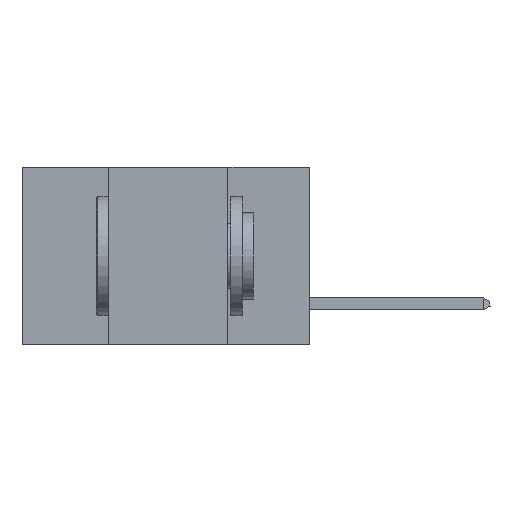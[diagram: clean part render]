
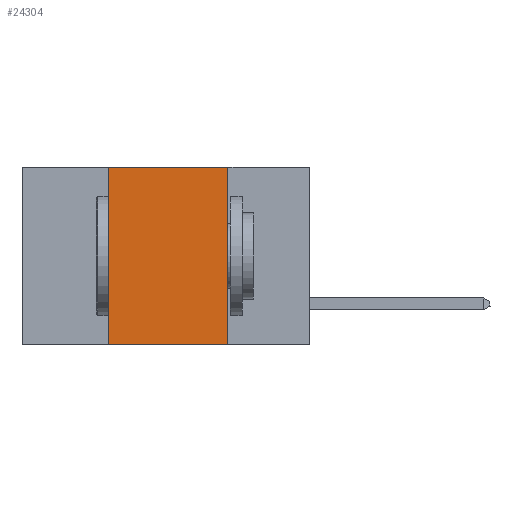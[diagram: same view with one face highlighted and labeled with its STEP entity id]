
A CAD part, left-side view. The second image highlights one B-rep face of the part: STEP entity #24304.
In plain terms, the highlighted planar face has unit normal (-1, 0, 0).
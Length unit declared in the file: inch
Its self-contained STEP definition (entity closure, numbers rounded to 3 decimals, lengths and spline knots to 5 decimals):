
#464 = AXIS2_PLACEMENT_3D ( 'NONE', #31716, #12325, #34604 ) ;
#1781 = ORIENTED_EDGE ( 'NONE', *, *, #29595, .T. ) ;
#3435 = VECTOR ( 'NONE', #9895, 39.37008 ) ;
#3680 = PLANE ( 'NONE',  #464 ) ;
#3790 = VERTEX_POINT ( 'NONE', #25234 ) ;
#9895 = DIRECTION ( 'NONE',  ( 0., -1., 0. ) ) ;
#10277 = LINE ( 'NONE', #16529, #36009 ) ;
#10820 = LINE ( 'NONE', #23432, #3435 ) ;
#10913 = ORIENTED_EDGE ( 'NONE', *, *, #31078, .F. ) ;
#11638 = LINE ( 'NONE', #31264, #20411 ) ;
#11940 = CARTESIAN_POINT ( 'NONE',  ( 0., 0.17, 0. ) ) ;
#12318 = VERTEX_POINT ( 'NONE', #19373 ) ;
#12325 = DIRECTION ( 'NONE',  ( 1., 0., 0. ) ) ;
#16529 = CARTESIAN_POINT ( 'NONE',  ( 0., 0.17, 0. ) ) ;
#16829 = EDGE_CURVE ( 'NONE', #3790, #17290, #10820, .T. ) ;
#16951 = CARTESIAN_POINT ( 'NONE',  ( 0., 0.42, -0.37 ) ) ;
#17148 = LINE ( 'NONE', #29473, #35852 ) ;
#17290 = VERTEX_POINT ( 'NONE', #11940 ) ;
#19373 = CARTESIAN_POINT ( 'NONE',  ( 0., 0.17, -0.37 ) ) ;
#20411 = VECTOR ( 'NONE', #25915, 39.37008 ) ;
#20912 = DIRECTION ( 'NONE',  ( 0., 0., 1. ) ) ;
#21212 = VERTEX_POINT ( 'NONE', #16951 ) ;
#23090 = DIRECTION ( 'NONE',  ( 0., 0., -1. ) ) ;
#23432 = CARTESIAN_POINT ( 'NONE',  ( 0., 0.6, 0. ) ) ;
#24286 = FACE_OUTER_BOUND ( 'NONE', #30659, .T. ) ;
#24304 = ADVANCED_FACE ( 'NONE', ( #24286 ), #3680, .F. ) ;
#25234 = CARTESIAN_POINT ( 'NONE',  ( 0., 0.42, 0. ) ) ;
#25915 = DIRECTION ( 'NONE',  ( 0., -1., 0. ) ) ;
#26725 = EDGE_CURVE ( 'NONE', #21212, #3790, #17148, .T. ) ;
#29473 = CARTESIAN_POINT ( 'NONE',  ( 0., 0.42, 0. ) ) ;
#29595 = EDGE_CURVE ( 'NONE', #21212, #12318, #11638, .T. ) ;
#30659 = EDGE_LOOP ( 'NONE', ( #10913, #32470, #31042, #1781 ) ) ;
#31042 = ORIENTED_EDGE ( 'NONE', *, *, #26725, .F. ) ;
#31078 = EDGE_CURVE ( 'NONE', #17290, #12318, #10277, .T. ) ;
#31264 = CARTESIAN_POINT ( 'NONE',  ( 0., 0.6, -0.37 ) ) ;
#31716 = CARTESIAN_POINT ( 'NONE',  ( 0., 0.6, 0. ) ) ;
#32470 = ORIENTED_EDGE ( 'NONE', *, *, #16829, .F. ) ;
#34604 = DIRECTION ( 'NONE',  ( 0., 0., -1. ) ) ;
#35852 = VECTOR ( 'NONE', #20912, 39.37008 ) ;
#36009 = VECTOR ( 'NONE', #23090, 39.37008 ) ;
